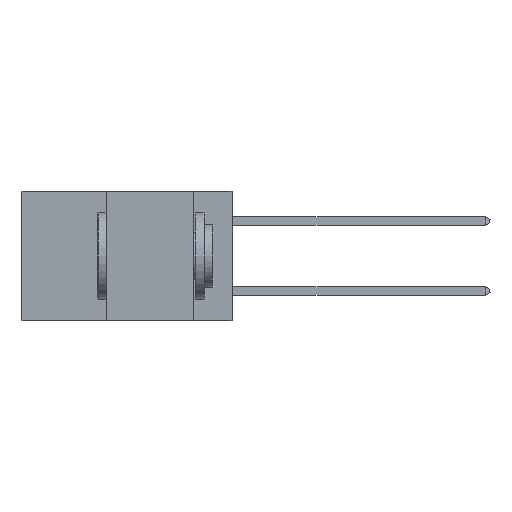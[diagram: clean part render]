
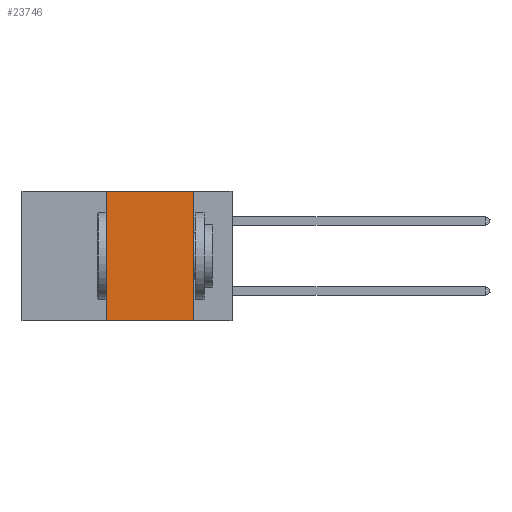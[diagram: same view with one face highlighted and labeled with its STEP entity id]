
A CAD part, left-side view. The second image highlights one B-rep face of the part: STEP entity #23746.
In plain terms, the highlighted planar face has unit normal (-1, 0, 0).
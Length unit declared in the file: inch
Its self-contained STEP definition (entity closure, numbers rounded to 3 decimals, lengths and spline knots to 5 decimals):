
#340 = CARTESIAN_POINT ( 'NONE',  ( 0., 0.36, -0.37 ) ) ;
#1709 = EDGE_CURVE ( 'NONE', #2245, #5119, #12188, .T. ) ;
#2245 = VERTEX_POINT ( 'NONE', #340 ) ;
#3916 = EDGE_LOOP ( 'NONE', ( #12218, #13802, #14992, #15322 ) ) ;
#4745 = VERTEX_POINT ( 'NONE', #6202 ) ;
#4836 = VECTOR ( 'NONE', #32878, 39.37008 ) ;
#5119 = VERTEX_POINT ( 'NONE', #15528 ) ;
#5967 = VECTOR ( 'NONE', #23127, 39.37008 ) ;
#6202 = CARTESIAN_POINT ( 'NONE',  ( 0., 0.11, 0. ) ) ;
#6610 = PLANE ( 'NONE',  #17113 ) ;
#6727 = DIRECTION ( 'NONE',  ( 0., 0., -1. ) ) ;
#8623 = VERTEX_POINT ( 'NONE', #13210 ) ;
#10677 = FACE_OUTER_BOUND ( 'NONE', #3916, .T. ) ;
#12188 = LINE ( 'NONE', #23458, #5967 ) ;
#12218 = ORIENTED_EDGE ( 'NONE', *, *, #15934, .F. ) ;
#13210 = CARTESIAN_POINT ( 'NONE',  ( 0., 0.11, -0.37 ) ) ;
#13802 = ORIENTED_EDGE ( 'NONE', *, *, #21148, .F. ) ;
#14497 = CARTESIAN_POINT ( 'NONE',  ( 0., 0.6, 0. ) ) ;
#14579 = CARTESIAN_POINT ( 'NONE',  ( 0., 0.6, 0. ) ) ;
#14710 = LINE ( 'NONE', #17622, #21582 ) ;
#14992 = ORIENTED_EDGE ( 'NONE', *, *, #1709, .F. ) ;
#15322 = ORIENTED_EDGE ( 'NONE', *, *, #27572, .T. ) ;
#15528 = CARTESIAN_POINT ( 'NONE',  ( 0., 0.36, 0. ) ) ;
#15934 = EDGE_CURVE ( 'NONE', #4745, #8623, #14710, .T. ) ;
#17113 = AXIS2_PLACEMENT_3D ( 'NONE', #14579, #22395, #6727 ) ;
#17622 = CARTESIAN_POINT ( 'NONE',  ( 0., 0.11, 0. ) ) ;
#17840 = LINE ( 'NONE', #14497, #30670 ) ;
#18862 = LINE ( 'NONE', #30348, #4836 ) ;
#20217 = DIRECTION ( 'NONE',  ( 0., 0., -1. ) ) ;
#21148 = EDGE_CURVE ( 'NONE', #5119, #4745, #17840, .T. ) ;
#21582 = VECTOR ( 'NONE', #20217, 39.37008 ) ;
#22395 = DIRECTION ( 'NONE',  ( 1., 0., 0. ) ) ;
#23127 = DIRECTION ( 'NONE',  ( 0., 0., 1. ) ) ;
#23458 = CARTESIAN_POINT ( 'NONE',  ( 0., 0.36, 0. ) ) ;
#23746 = ADVANCED_FACE ( 'NONE', ( #10677 ), #6610, .F. ) ;
#27572 = EDGE_CURVE ( 'NONE', #2245, #8623, #18862, .T. ) ;
#30052 = DIRECTION ( 'NONE',  ( 0., -1., 0. ) ) ;
#30348 = CARTESIAN_POINT ( 'NONE',  ( 0., 0.6, -0.37 ) ) ;
#30670 = VECTOR ( 'NONE', #30052, 39.37008 ) ;
#32878 = DIRECTION ( 'NONE',  ( 0., -1., 0. ) ) ;
